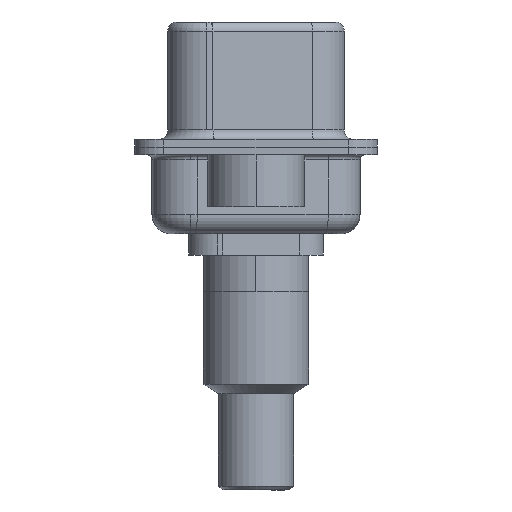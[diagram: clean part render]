
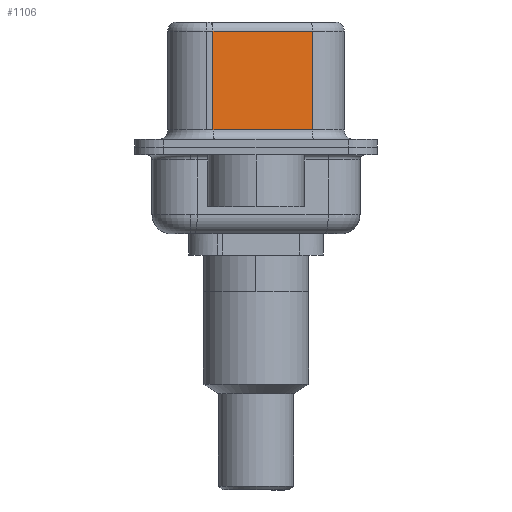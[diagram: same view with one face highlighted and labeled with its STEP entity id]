
A CAD part, left-side view. The second image highlights one B-rep face of the part: STEP entity #1106.
In plain terms, the highlighted planar face has unit normal (-0.985, -0.174, 0).
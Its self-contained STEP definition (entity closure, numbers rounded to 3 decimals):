
#239 = DIRECTION ( 'NONE',  ( 0., 0., -1. ) ) ;
#592 = CARTESIAN_POINT ( 'NONE',  ( 3.67, 2.233, 6.02 ) ) ;
#1021 = AXIS2_PLACEMENT_3D ( 'NONE', #18638, #14696, #14776 ) ;
#1106 = ADVANCED_FACE ( 'NONE', ( #12919 ), #16794, .F. ) ;
#1881 = DIRECTION ( 'NONE',  ( 0.174, -0.985, 0. ) ) ;
#3756 = ORIENTED_EDGE ( 'NONE', *, *, #19735, .T. ) ;
#5693 = VERTEX_POINT ( 'NONE', #22979 ) ;
#5841 = VECTOR ( 'NONE', #9197, 1000. ) ;
#6477 = LINE ( 'NONE', #11293, #5841 ) ;
#8993 = ORIENTED_EDGE ( 'NONE', *, *, #21066, .F. ) ;
#9197 = DIRECTION ( 'NONE',  ( 0., 0., -1. ) ) ;
#9469 = VERTEX_POINT ( 'NONE', #11600 ) ;
#9789 = CARTESIAN_POINT ( 'NONE',  ( 4.58, -2.927, 6.02 ) ) ;
#11033 = LINE ( 'NONE', #20002, #15770 ) ;
#11293 = CARTESIAN_POINT ( 'NONE',  ( 3.67, 2.233, 6.52 ) ) ;
#11600 = CARTESIAN_POINT ( 'NONE',  ( 4.58, -2.927, 6.02 ) ) ;
#12127 = ORIENTED_EDGE ( 'NONE', *, *, #23688, .T. ) ;
#12919 = FACE_OUTER_BOUND ( 'NONE', #23042, .T. ) ;
#13409 = VECTOR ( 'NONE', #23849, 1000. ) ;
#14033 = LINE ( 'NONE', #9789, #13409 ) ;
#14696 = DIRECTION ( 'NONE',  ( 0.985, 0.174, 0. ) ) ;
#14776 = DIRECTION ( 'NONE',  ( -0.174, 0.985, 0. ) ) ;
#15770 = VECTOR ( 'NONE', #1881, 1000. ) ;
#16794 = PLANE ( 'NONE',  #1021 ) ;
#18638 = CARTESIAN_POINT ( 'NONE',  ( 4.58, -2.927, 6.52 ) ) ;
#18938 = VECTOR ( 'NONE', #239, 1000. ) ;
#19735 = EDGE_CURVE ( 'NONE', #5693, #23247, #11033, .T. ) ;
#20002 = CARTESIAN_POINT ( 'NONE',  ( 4.58, -2.927, 0.9 ) ) ;
#20409 = ORIENTED_EDGE ( 'NONE', *, *, #23829, .T. ) ;
#21066 = EDGE_CURVE ( 'NONE', #9469, #23247, #24837, .T. ) ;
#21181 = VERTEX_POINT ( 'NONE', #592 ) ;
#22979 = CARTESIAN_POINT ( 'NONE',  ( 3.67, 2.233, 0.9 ) ) ;
#23042 = EDGE_LOOP ( 'NONE', ( #8993, #20409, #12127, #3756 ) ) ;
#23247 = VERTEX_POINT ( 'NONE', #25964 ) ;
#23688 = EDGE_CURVE ( 'NONE', #21181, #5693, #6477, .T. ) ;
#23829 = EDGE_CURVE ( 'NONE', #9469, #21181, #14033, .T. ) ;
#23849 = DIRECTION ( 'NONE',  ( -0.174, 0.985, 0. ) ) ;
#24373 = CARTESIAN_POINT ( 'NONE',  ( 4.58, -2.927, 6.52 ) ) ;
#24837 = LINE ( 'NONE', #24373, #18938 ) ;
#25964 = CARTESIAN_POINT ( 'NONE',  ( 4.58, -2.927, 0.9 ) ) ;
